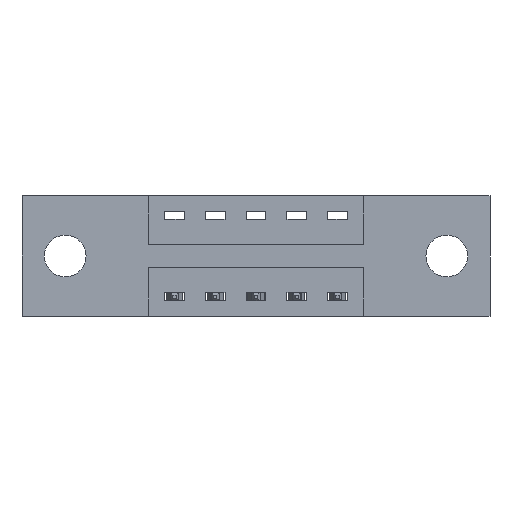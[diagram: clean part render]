
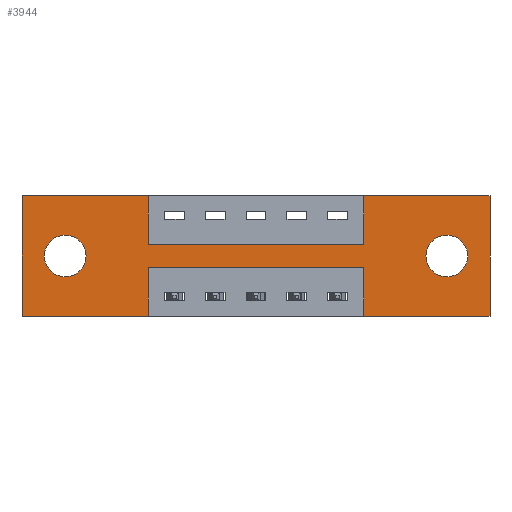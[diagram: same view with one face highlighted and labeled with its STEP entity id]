
A CAD part, front view. The second image highlights one B-rep face of the part: STEP entity #3944.
In plain terms, the highlighted planar face has unit normal (0, -1, 0).
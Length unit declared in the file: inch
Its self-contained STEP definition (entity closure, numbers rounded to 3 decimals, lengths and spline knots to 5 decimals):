
#105 = EDGE_CURVE ( 'NONE', #3751, #1631, #4860, .T. ) ;
#106 = CARTESIAN_POINT ( 'NONE',  ( 0.3875, 0., -0.15 ) ) ;
#193 = EDGE_CURVE ( 'NONE', #1631, #4997, #3957, .T. ) ;
#269 = LINE ( 'NONE', #3084, #2325 ) ;
#308 = VECTOR ( 'NONE', #799, 39.37008 ) ;
#318 = DIRECTION ( 'NONE',  ( 0., 0., -1. ) ) ;
#340 = DIRECTION ( 'NONE',  ( -1., 0., 0. ) ) ;
#495 = ORIENTED_EDGE ( 'NONE', *, *, #6731, .F. ) ;
#560 = LINE ( 'NONE', #2836, #2578 ) ;
#588 = AXIS2_PLACEMENT_3D ( 'NONE', #4838, #1090, #1739 ) ;
#646 = CARTESIAN_POINT ( 'NONE',  ( 0., 0., 0. ) ) ;
#799 = DIRECTION ( 'NONE',  ( 0., 0., -1. ) ) ;
#814 = VECTOR ( 'NONE', #3913, 39.37008 ) ;
#834 = AXIS2_PLACEMENT_3D ( 'NONE', #2866, #1025, #2276 ) ;
#864 = CARTESIAN_POINT ( 'NONE',  ( 0., 0., 0. ) ) ;
#896 = CARTESIAN_POINT ( 'NONE',  ( 1.0475, 0., -0.37 ) ) ;
#949 = CARTESIAN_POINT ( 'NONE',  ( 0.3875, 0., -0.37 ) ) ;
#959 = CARTESIAN_POINT ( 'NONE',  ( 0.3875, 0., -0.22 ) ) ;
#1025 = DIRECTION ( 'NONE',  ( 0., -1., 0. ) ) ;
#1080 = EDGE_CURVE ( 'NONE', #6763, #7095, #7952, .T. ) ;
#1090 = DIRECTION ( 'NONE',  ( 0., 1., 0. ) ) ;
#1156 = EDGE_CURVE ( 'NONE', #7095, #5632, #5761, .T. ) ;
#1188 = DIRECTION ( 'NONE',  ( 0., 0., 1. ) ) ;
#1215 = ORIENTED_EDGE ( 'NONE', *, *, #7609, .F. ) ;
#1224 = AXIS2_PLACEMENT_3D ( 'NONE', #4736, #4089, #318 ) ;
#1258 = ORIENTED_EDGE ( 'NONE', *, *, #1080, .F. ) ;
#1293 = VERTEX_POINT ( 'NONE', #8028 ) ;
#1397 = VECTOR ( 'NONE', #4054, 39.37008 ) ;
#1451 = EDGE_CURVE ( 'NONE', #3745, #2398, #1703, .T. ) ;
#1562 = CARTESIAN_POINT ( 'NONE',  ( 1.0475, 0., 0. ) ) ;
#1566 = EDGE_CURVE ( 'NONE', #4997, #6763, #6612, .T. ) ;
#1571 = CARTESIAN_POINT ( 'NONE',  ( 0., 0., 0. ) ) ;
#1594 = PLANE ( 'NONE',  #834 ) ;
#1631 = VERTEX_POINT ( 'NONE', #4572 ) ;
#1637 = CARTESIAN_POINT ( 'NONE',  ( 1.0475, 0., -0.22 ) ) ;
#1651 = VERTEX_POINT ( 'NONE', #5975 ) ;
#1702 = CIRCLE ( 'NONE', #3270, 0.064 ) ;
#1703 = LINE ( 'NONE', #7851, #7420 ) ;
#1736 = ORIENTED_EDGE ( 'NONE', *, *, #6510, .F. ) ;
#1739 = DIRECTION ( 'NONE',  ( 0., 0., -1. ) ) ;
#1882 = CARTESIAN_POINT ( 'NONE',  ( 0.1325, 0., -0.249 ) ) ;
#2064 = VECTOR ( 'NONE', #3646, 39.37008 ) ;
#2193 = EDGE_CURVE ( 'NONE', #7991, #4381, #6761, .T. ) ;
#2276 = DIRECTION ( 'NONE',  ( 0., 0., -1. ) ) ;
#2325 = VECTOR ( 'NONE', #4969, 39.37008 ) ;
#2398 = VERTEX_POINT ( 'NONE', #959 ) ;
#2578 = VECTOR ( 'NONE', #5991, 39.37008 ) ;
#2600 = DIRECTION ( 'NONE',  ( 1., 0., 0. ) ) ;
#2775 = LINE ( 'NONE', #1562, #1397 ) ;
#2836 = CARTESIAN_POINT ( 'NONE',  ( 0., 0., -0.37 ) ) ;
#2864 = DIRECTION ( 'NONE',  ( 0., 1., 0. ) ) ;
#2866 = CARTESIAN_POINT ( 'NONE',  ( 0., 0., -0.37 ) ) ;
#2900 = CARTESIAN_POINT ( 'NONE',  ( 0.3875, 0., -0.15 ) ) ;
#2998 = ORIENTED_EDGE ( 'NONE', *, *, #5511, .T. ) ;
#3010 = CARTESIAN_POINT ( 'NONE',  ( 1.435, 0., 0. ) ) ;
#3035 = CARTESIAN_POINT ( 'NONE',  ( 0.3875, 0., 0. ) ) ;
#3065 = VECTOR ( 'NONE', #2600, 39.37008 ) ;
#3084 = CARTESIAN_POINT ( 'NONE',  ( 1.0475, 0., -0.37 ) ) ;
#3110 = EDGE_CURVE ( 'NONE', #3281, #1293, #3826, .T. ) ;
#3165 = VERTEX_POINT ( 'NONE', #896 ) ;
#3208 = AXIS2_PLACEMENT_3D ( 'NONE', #5281, #4273, #1188 ) ;
#3270 = AXIS2_PLACEMENT_3D ( 'NONE', #4084, #2864, #4650 ) ;
#3281 = VERTEX_POINT ( 'NONE', #4955 ) ;
#3305 = DIRECTION ( 'NONE',  ( -1., 0., 0. ) ) ;
#3373 = VERTEX_POINT ( 'NONE', #7635 ) ;
#3483 = CARTESIAN_POINT ( 'NONE',  ( 0., 0., 0. ) ) ;
#3557 = ORIENTED_EDGE ( 'NONE', *, *, #1451, .F. ) ;
#3596 = EDGE_LOOP ( 'NONE', ( #3891, #4314 ) ) ;
#3646 = DIRECTION ( 'NONE',  ( 0., 0., -1. ) ) ;
#3745 = VERTEX_POINT ( 'NONE', #1637 ) ;
#3751 = VERTEX_POINT ( 'NONE', #949 ) ;
#3764 = ORIENTED_EDGE ( 'NONE', *, *, #6730, .T. ) ;
#3826 = LINE ( 'NONE', #646, #3065 ) ;
#3891 = ORIENTED_EDGE ( 'NONE', *, *, #2193, .T. ) ;
#3913 = DIRECTION ( 'NONE',  ( 1., 0., 0. ) ) ;
#3944 = ADVANCED_FACE ( 'NONE', ( #5276, #7190, #7895 ), #1594, .T. ) ;
#3957 = LINE ( 'NONE', #864, #4029 ) ;
#4029 = VECTOR ( 'NONE', #6013, 39.37008 ) ;
#4054 = DIRECTION ( 'NONE',  ( 0., 0., 1. ) ) ;
#4084 = CARTESIAN_POINT ( 'NONE',  ( 0.1325, 0., -0.185 ) ) ;
#4089 = DIRECTION ( 'NONE',  ( 0., 1., 0. ) ) ;
#4216 = LINE ( 'NONE', #3010, #2064 ) ;
#4268 = CARTESIAN_POINT ( 'NONE',  ( 0.3875, 0., 0. ) ) ;
#4273 = DIRECTION ( 'NONE',  ( 0., 1., 0. ) ) ;
#4314 = ORIENTED_EDGE ( 'NONE', *, *, #5103, .T. ) ;
#4381 = VERTEX_POINT ( 'NONE', #1882 ) ;
#4572 = CARTESIAN_POINT ( 'NONE',  ( 0., 0., -0.37 ) ) ;
#4650 = DIRECTION ( 'NONE',  ( 0., 0., 1. ) ) ;
#4731 = CARTESIAN_POINT ( 'NONE',  ( 0.1325, 0., -0.121 ) ) ;
#4736 = CARTESIAN_POINT ( 'NONE',  ( 1.3025, 0., -0.185 ) ) ;
#4838 = CARTESIAN_POINT ( 'NONE',  ( 1.3025, 0., -0.185 ) ) ;
#4860 = LINE ( 'NONE', #7398, #7701 ) ;
#4884 = VECTOR ( 'NONE', #8118, 39.37008 ) ;
#4886 = ORIENTED_EDGE ( 'NONE', *, *, #193, .F. ) ;
#4887 = CARTESIAN_POINT ( 'NONE',  ( 1.0475, 0., -0.15 ) ) ;
#4894 = CIRCLE ( 'NONE', #1224, 0.064 ) ;
#4955 = CARTESIAN_POINT ( 'NONE',  ( 1.0475, 0., 0. ) ) ;
#4969 = DIRECTION ( 'NONE',  ( 0., 0., 1. ) ) ;
#4997 = VERTEX_POINT ( 'NONE', #1571 ) ;
#5103 = EDGE_CURVE ( 'NONE', #4381, #7991, #1702, .T. ) ;
#5113 = EDGE_LOOP ( 'NONE', ( #3764, #2998 ) ) ;
#5120 = CARTESIAN_POINT ( 'NONE',  ( 1.3025, 0., -0.249 ) ) ;
#5223 = ORIENTED_EDGE ( 'NONE', *, *, #105, .F. ) ;
#5276 = FACE_BOUND ( 'NONE', #5113, .T. ) ;
#5281 = CARTESIAN_POINT ( 'NONE',  ( 0.1325, 0., -0.185 ) ) ;
#5511 = EDGE_CURVE ( 'NONE', #7723, #3373, #4894, .T. ) ;
#5632 = VERTEX_POINT ( 'NONE', #4887 ) ;
#5761 = LINE ( 'NONE', #106, #814 ) ;
#5953 = VECTOR ( 'NONE', #7114, 39.37008 ) ;
#5975 = CARTESIAN_POINT ( 'NONE',  ( 1.435, 0., -0.37 ) ) ;
#5991 = DIRECTION ( 'NONE',  ( -1., 0., 0. ) ) ;
#5999 = ORIENTED_EDGE ( 'NONE', *, *, #1156, .F. ) ;
#6013 = DIRECTION ( 'NONE',  ( 0., 0., 1. ) ) ;
#6296 = EDGE_CURVE ( 'NONE', #5632, #3281, #2775, .T. ) ;
#6407 = CIRCLE ( 'NONE', #588, 0.064 ) ;
#6510 = EDGE_CURVE ( 'NONE', #3165, #3745, #269, .T. ) ;
#6546 = LINE ( 'NONE', #7212, #308 ) ;
#6612 = LINE ( 'NONE', #3483, #5953 ) ;
#6730 = EDGE_CURVE ( 'NONE', #3373, #7723, #6407, .T. ) ;
#6731 = EDGE_CURVE ( 'NONE', #1293, #1651, #4216, .T. ) ;
#6761 = CIRCLE ( 'NONE', #3208, 0.064 ) ;
#6763 = VERTEX_POINT ( 'NONE', #3035 ) ;
#6922 = EDGE_CURVE ( 'NONE', #1651, #3165, #560, .T. ) ;
#7095 = VERTEX_POINT ( 'NONE', #2900 ) ;
#7114 = DIRECTION ( 'NONE',  ( 1., 0., 0. ) ) ;
#7158 = ORIENTED_EDGE ( 'NONE', *, *, #6296, .F. ) ;
#7190 = FACE_BOUND ( 'NONE', #3596, .T. ) ;
#7211 = ORIENTED_EDGE ( 'NONE', *, *, #1566, .F. ) ;
#7212 = CARTESIAN_POINT ( 'NONE',  ( 0.3875, 0., -0.37 ) ) ;
#7398 = CARTESIAN_POINT ( 'NONE',  ( 0., 0., -0.37 ) ) ;
#7419 = ORIENTED_EDGE ( 'NONE', *, *, #3110, .F. ) ;
#7420 = VECTOR ( 'NONE', #340, 39.37008 ) ;
#7449 = EDGE_LOOP ( 'NONE', ( #1215, #3557, #1736, #7951, #495, #7419, #7158, #5999, #1258, #7211, #4886, #5223 ) ) ;
#7609 = EDGE_CURVE ( 'NONE', #2398, #3751, #6546, .T. ) ;
#7635 = CARTESIAN_POINT ( 'NONE',  ( 1.3025, 0., -0.121 ) ) ;
#7701 = VECTOR ( 'NONE', #3305, 39.37008 ) ;
#7723 = VERTEX_POINT ( 'NONE', #5120 ) ;
#7851 = CARTESIAN_POINT ( 'NONE',  ( 0.3875, 0., -0.22 ) ) ;
#7895 = FACE_OUTER_BOUND ( 'NONE', #7449, .T. ) ;
#7951 = ORIENTED_EDGE ( 'NONE', *, *, #6922, .F. ) ;
#7952 = LINE ( 'NONE', #4268, #4884 ) ;
#7991 = VERTEX_POINT ( 'NONE', #4731 ) ;
#8028 = CARTESIAN_POINT ( 'NONE',  ( 1.435, 0., 0. ) ) ;
#8118 = DIRECTION ( 'NONE',  ( 0., 0., -1. ) ) ;
